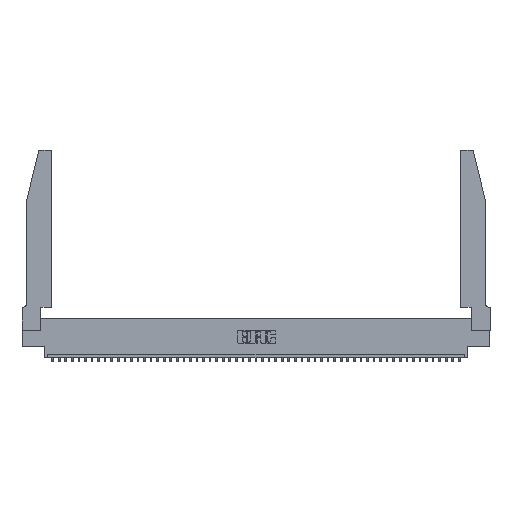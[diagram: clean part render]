
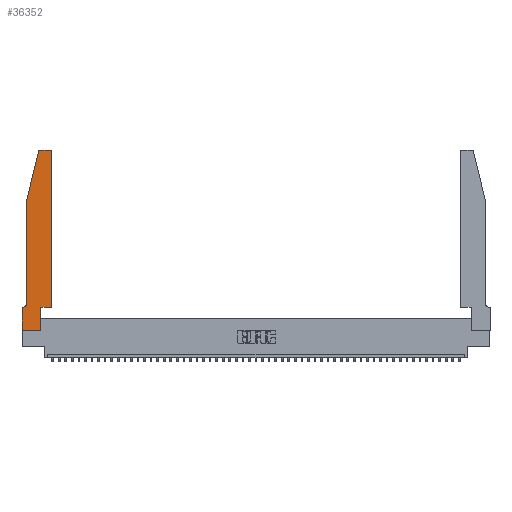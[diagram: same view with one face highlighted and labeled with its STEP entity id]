
A CAD part, top view. The second image highlights one B-rep face of the part: STEP entity #36352.
In plain terms, the highlighted planar face has unit normal (0, 0, 1).
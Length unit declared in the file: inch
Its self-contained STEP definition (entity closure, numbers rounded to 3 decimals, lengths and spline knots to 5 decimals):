
#481 = EDGE_CURVE ( 'NONE', #23314, #12050, #9472, .T. ) ;
#530 = CARTESIAN_POINT ( 'NONE',  ( 0., 0., 0.37 ) ) ;
#941 = EDGE_CURVE ( 'NONE', #4561, #31325, #45455, .T. ) ;
#2247 = ORIENTED_EDGE ( 'NONE', *, *, #16603, .T. ) ;
#2322 = CARTESIAN_POINT ( 'NONE',  ( 0., 0., 0.37 ) ) ;
#3190 = LINE ( 'NONE', #18290, #42712 ) ;
#3651 = EDGE_CURVE ( 'NONE', #12050, #12766, #7420, .T. ) ;
#4122 = EDGE_CURVE ( 'NONE', #12766, #38531, #48700, .T. ) ;
#4561 = VERTEX_POINT ( 'NONE', #2322 ) ;
#5264 = VECTOR ( 'NONE', #11345, 39.37008 ) ;
#5797 = VERTEX_POINT ( 'NONE', #44779 ) ;
#5899 = VERTEX_POINT ( 'NONE', #31076 ) ;
#7420 = CIRCLE ( 'NONE', #8970, 0.03 ) ;
#8423 = ORIENTED_EDGE ( 'NONE', *, *, #4122, .T. ) ;
#8723 = DIRECTION ( 'NONE',  ( 0., -1., 0. ) ) ;
#8970 = AXIS2_PLACEMENT_3D ( 'NONE', #24104, #21614, #42662 ) ;
#9051 = ORIENTED_EDGE ( 'NONE', *, *, #941, .T. ) ;
#9472 = LINE ( 'NONE', #46335, #5264 ) ;
#9640 = EDGE_CURVE ( 'NONE', #5797, #4561, #26376, .T. ) ;
#9650 = VERTEX_POINT ( 'NONE', #20661 ) ;
#10746 = CARTESIAN_POINT ( 'NONE',  ( 0.2865, 0.35, 0.37 ) ) ;
#10940 = VECTOR ( 'NONE', #26403, 39.37008 ) ;
#11345 = DIRECTION ( 'NONE',  ( -1., 0., 0. ) ) ;
#11946 = CARTESIAN_POINT ( 'NONE',  ( 0.0755, 2., 0.37 ) ) ;
#12050 = VERTEX_POINT ( 'NONE', #36200 ) ;
#12766 = VERTEX_POINT ( 'NONE', #12892 ) ;
#12798 = CARTESIAN_POINT ( 'NONE',  ( 0.4505, 0.35, 0.37 ) ) ;
#12892 = CARTESIAN_POINT ( 'NONE',  ( 0.25487, 2.72718, 0.37 ) ) ;
#14397 = DIRECTION ( 'NONE',  ( -1., 0., 0. ) ) ;
#14562 = DIRECTION ( 'NONE',  ( 0., 1., 0. ) ) ;
#14979 = VECTOR ( 'NONE', #31771, 39.37008 ) ;
#15033 = PLANE ( 'NONE',  #23467 ) ;
#15796 = ORIENTED_EDGE ( 'NONE', *, *, #481, .T. ) ;
#16181 = ORIENTED_EDGE ( 'NONE', *, *, #18800, .T. ) ;
#16603 = EDGE_CURVE ( 'NONE', #5899, #23925, #38433, .T. ) ;
#17154 = ORIENTED_EDGE ( 'NONE', *, *, #9640, .T. ) ;
#17329 = LINE ( 'NONE', #29244, #49103 ) ;
#17352 = DIRECTION ( 'NONE',  ( 0., -1., 0. ) ) ;
#17599 = DIRECTION ( 'NONE',  ( -1., 0., 0. ) ) ;
#18290 = CARTESIAN_POINT ( 'NONE',  ( 0.0755, 0.35, 0.37 ) ) ;
#18475 = LINE ( 'NONE', #47885, #35176 ) ;
#18800 = EDGE_CURVE ( 'NONE', #31325, #26231, #18475, .T. ) ;
#19495 = CARTESIAN_POINT ( 'NONE',  ( 0., 0., 0.37 ) ) ;
#20180 = DIRECTION ( 'NONE',  ( 1., 0., 0. ) ) ;
#20510 = CARTESIAN_POINT ( 'NONE',  ( 0.4505, 2.72, 0.37 ) ) ;
#20661 = CARTESIAN_POINT ( 'NONE',  ( 0.0755, 0.42, 0.37 ) ) ;
#21614 = DIRECTION ( 'NONE',  ( 0., 0., 1. ) ) ;
#21767 = CARTESIAN_POINT ( 'NONE',  ( 0.0055, 0.35, 0.37 ) ) ;
#23153 = AXIS2_PLACEMENT_3D ( 'NONE', #44931, #25495, #14397 ) ;
#23314 = VERTEX_POINT ( 'NONE', #36503 ) ;
#23361 = EDGE_CURVE ( 'NONE', #38531, #9650, #17329, .T. ) ;
#23467 = AXIS2_PLACEMENT_3D ( 'NONE', #41885, #42040, #45861 ) ;
#23680 = DIRECTION ( 'NONE',  ( 1., 0., 0. ) ) ;
#23827 = ORIENTED_EDGE ( 'NONE', *, *, #23361, .T. ) ;
#23851 = DIRECTION ( 'NONE',  ( 0., 0., 1. ) ) ;
#23925 = VERTEX_POINT ( 'NONE', #20510 ) ;
#24104 = CARTESIAN_POINT ( 'NONE',  ( 0.284, 2.72, 0.37 ) ) ;
#24259 = ORIENTED_EDGE ( 'NONE', *, *, #34586, .T. ) ;
#24518 = CARTESIAN_POINT ( 'NONE',  ( 0.0755, 2., 0.37 ) ) ;
#24805 = EDGE_LOOP ( 'NONE', ( #15796, #46578, #8423, #23827, #24259, #35782, #17154, #9051, #16181, #26744, #2247, #27152 ) ) ;
#25495 = DIRECTION ( 'NONE',  ( 0., 0., -1. ) ) ;
#25569 = VERTEX_POINT ( 'NONE', #21767 ) ;
#26231 = VERTEX_POINT ( 'NONE', #10746 ) ;
#26376 = LINE ( 'NONE', #19495, #32937 ) ;
#26403 = DIRECTION ( 'NONE',  ( -0.239, -0.971, 0. ) ) ;
#26614 = LINE ( 'NONE', #33981, #45776 ) ;
#26744 = ORIENTED_EDGE ( 'NONE', *, *, #35740, .T. ) ;
#27152 = ORIENTED_EDGE ( 'NONE', *, *, #49398, .T. ) ;
#27364 = CARTESIAN_POINT ( 'NONE',  ( 0.4205, 2.72, 0.37 ) ) ;
#29244 = CARTESIAN_POINT ( 'NONE',  ( 0.0755, 2., 0.37 ) ) ;
#31076 = CARTESIAN_POINT ( 'NONE',  ( 0.4505, 0.35, 0.37 ) ) ;
#31325 = VERTEX_POINT ( 'NONE', #42641 ) ;
#31771 = DIRECTION ( 'NONE',  ( 0., 1., 0. ) ) ;
#31990 = CIRCLE ( 'NONE', #35719, 0.03 ) ;
#32937 = VECTOR ( 'NONE', #17352, 39.37008 ) ;
#33981 = CARTESIAN_POINT ( 'NONE',  ( 0.4505, 0.35, 0.37 ) ) ;
#34586 = EDGE_CURVE ( 'NONE', #9650, #25569, #42307, .T. ) ;
#35176 = VECTOR ( 'NONE', #14562, 39.37008 ) ;
#35719 = AXIS2_PLACEMENT_3D ( 'NONE', #27364, #23851, #23680 ) ;
#35740 = EDGE_CURVE ( 'NONE', #26231, #5899, #26614, .T. ) ;
#35782 = ORIENTED_EDGE ( 'NONE', *, *, #44355, .T. ) ;
#36200 = CARTESIAN_POINT ( 'NONE',  ( 0.284, 2.75, 0.37 ) ) ;
#36352 = ADVANCED_FACE ( 'NONE', ( #40353 ), #15033, .T. ) ;
#36503 = CARTESIAN_POINT ( 'NONE',  ( 0.4205, 2.75, 0.37 ) ) ;
#38433 = LINE ( 'NONE', #12798, #14979 ) ;
#38531 = VERTEX_POINT ( 'NONE', #11946 ) ;
#40353 = FACE_OUTER_BOUND ( 'NONE', #24805, .T. ) ;
#41885 = CARTESIAN_POINT ( 'NONE',  ( 0., 0.35, 0.37 ) ) ;
#41992 = DIRECTION ( 'NONE',  ( 1., 0., 0. ) ) ;
#42040 = DIRECTION ( 'NONE',  ( 0., 0., 1. ) ) ;
#42307 = CIRCLE ( 'NONE', #23153, 0.07 ) ;
#42641 = CARTESIAN_POINT ( 'NONE',  ( 0.2865, 0., 0.37 ) ) ;
#42662 = DIRECTION ( 'NONE',  ( 1., 0., 0. ) ) ;
#42712 = VECTOR ( 'NONE', #17599, 39.37008 ) ;
#44355 = EDGE_CURVE ( 'NONE', #25569, #5797, #3190, .T. ) ;
#44779 = CARTESIAN_POINT ( 'NONE',  ( 0., 0.35, 0.37 ) ) ;
#44888 = VECTOR ( 'NONE', #20180, 39.37008 ) ;
#44931 = CARTESIAN_POINT ( 'NONE',  ( 0.0055, 0.42, 0.37 ) ) ;
#45455 = LINE ( 'NONE', #530, #44888 ) ;
#45776 = VECTOR ( 'NONE', #41992, 39.37008 ) ;
#45861 = DIRECTION ( 'NONE',  ( 1., 0., 0. ) ) ;
#46335 = CARTESIAN_POINT ( 'NONE',  ( 0.2605, 2.75, 0.37 ) ) ;
#46578 = ORIENTED_EDGE ( 'NONE', *, *, #3651, .T. ) ;
#47885 = CARTESIAN_POINT ( 'NONE',  ( 0.2865, 0.35, 0.37 ) ) ;
#48700 = LINE ( 'NONE', #24518, #10940 ) ;
#49103 = VECTOR ( 'NONE', #8723, 39.37008 ) ;
#49398 = EDGE_CURVE ( 'NONE', #23925, #23314, #31990, .T. ) ;
